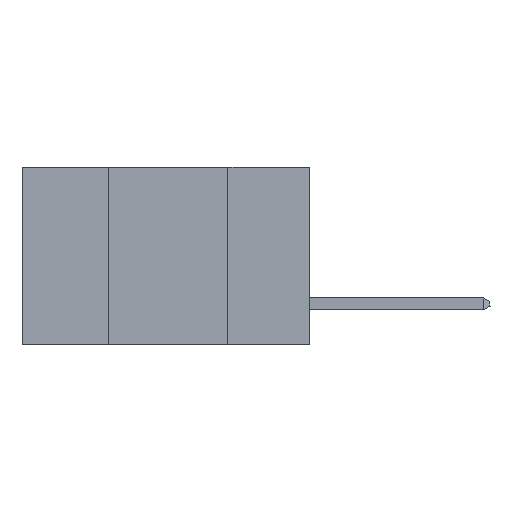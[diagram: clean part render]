
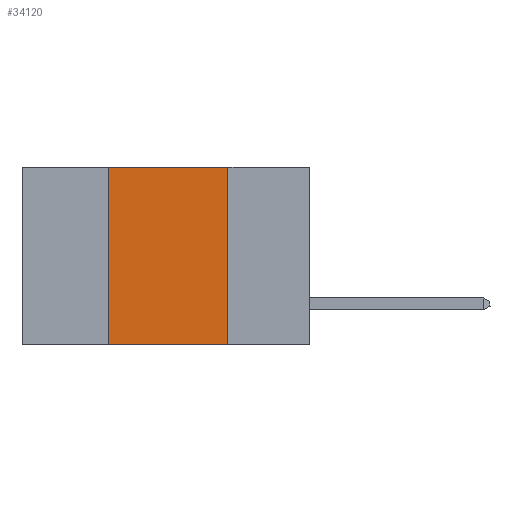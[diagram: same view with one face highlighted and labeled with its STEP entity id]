
A CAD part, left-side view. The second image highlights one B-rep face of the part: STEP entity #34120.
In plain terms, the highlighted planar face has unit normal (-1, 0, 0).
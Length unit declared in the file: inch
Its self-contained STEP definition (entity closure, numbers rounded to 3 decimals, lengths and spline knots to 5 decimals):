
#271 = CARTESIAN_POINT ( 'NONE',  ( 0., 0.42, -0.37 ) ) ;
#2294 = DIRECTION ( 'NONE',  ( 0., -1., 0. ) ) ;
#2688 = DIRECTION ( 'NONE',  ( 0., -1., 0. ) ) ;
#4408 = ORIENTED_EDGE ( 'NONE', *, *, #45690, .F. ) ;
#5705 = DIRECTION ( 'NONE',  ( 0., 0., 1. ) ) ;
#6944 = VECTOR ( 'NONE', #27415, 39.37008 ) ;
#9151 = CARTESIAN_POINT ( 'NONE',  ( 0., 0.6, 0. ) ) ;
#9610 = EDGE_CURVE ( 'NONE', #41752, #9739, #9617, .T. ) ;
#9617 = LINE ( 'NONE', #9151, #48252 ) ;
#9739 = VERTEX_POINT ( 'NONE', #20402 ) ;
#10212 = CARTESIAN_POINT ( 'NONE',  ( 0., 0.6, -0.37 ) ) ;
#11441 = DIRECTION ( 'NONE',  ( 0., 0., -1. ) ) ;
#11982 = VECTOR ( 'NONE', #5705, 39.37008 ) ;
#15431 = VECTOR ( 'NONE', #2294, 39.37008 ) ;
#15681 = EDGE_CURVE ( 'NONE', #46910, #21017, #36840, .T. ) ;
#16484 = ORIENTED_EDGE ( 'NONE', *, *, #9610, .F. ) ;
#17258 = ORIENTED_EDGE ( 'NONE', *, *, #38211, .F. ) ;
#20402 = CARTESIAN_POINT ( 'NONE',  ( 0., 0.17, 0. ) ) ;
#21017 = VERTEX_POINT ( 'NONE', #29867 ) ;
#22142 = AXIS2_PLACEMENT_3D ( 'NONE', #26754, #34200, #11441 ) ;
#22644 = EDGE_LOOP ( 'NONE', ( #17258, #16484, #4408, #48344 ) ) ;
#25725 = LINE ( 'NONE', #47733, #11982 ) ;
#26754 = CARTESIAN_POINT ( 'NONE',  ( 0., 0.6, 0. ) ) ;
#27415 = DIRECTION ( 'NONE',  ( 0., 0., -1. ) ) ;
#29867 = CARTESIAN_POINT ( 'NONE',  ( 0., 0.17, -0.37 ) ) ;
#34120 = ADVANCED_FACE ( 'NONE', ( #36616 ), #42013, .F. ) ;
#34200 = DIRECTION ( 'NONE',  ( 1., 0., 0. ) ) ;
#34696 = CARTESIAN_POINT ( 'NONE',  ( 0., 0.17, 0. ) ) ;
#36616 = FACE_OUTER_BOUND ( 'NONE', #22644, .T. ) ;
#36840 = LINE ( 'NONE', #10212, #15431 ) ;
#38211 = EDGE_CURVE ( 'NONE', #9739, #21017, #45023, .T. ) ;
#41752 = VERTEX_POINT ( 'NONE', #44643 ) ;
#42013 = PLANE ( 'NONE',  #22142 ) ;
#44643 = CARTESIAN_POINT ( 'NONE',  ( 0., 0.42, 0. ) ) ;
#45023 = LINE ( 'NONE', #34696, #6944 ) ;
#45690 = EDGE_CURVE ( 'NONE', #46910, #41752, #25725, .T. ) ;
#46910 = VERTEX_POINT ( 'NONE', #271 ) ;
#47733 = CARTESIAN_POINT ( 'NONE',  ( 0., 0.42, 0. ) ) ;
#48252 = VECTOR ( 'NONE', #2688, 39.37008 ) ;
#48344 = ORIENTED_EDGE ( 'NONE', *, *, #15681, .T. ) ;
